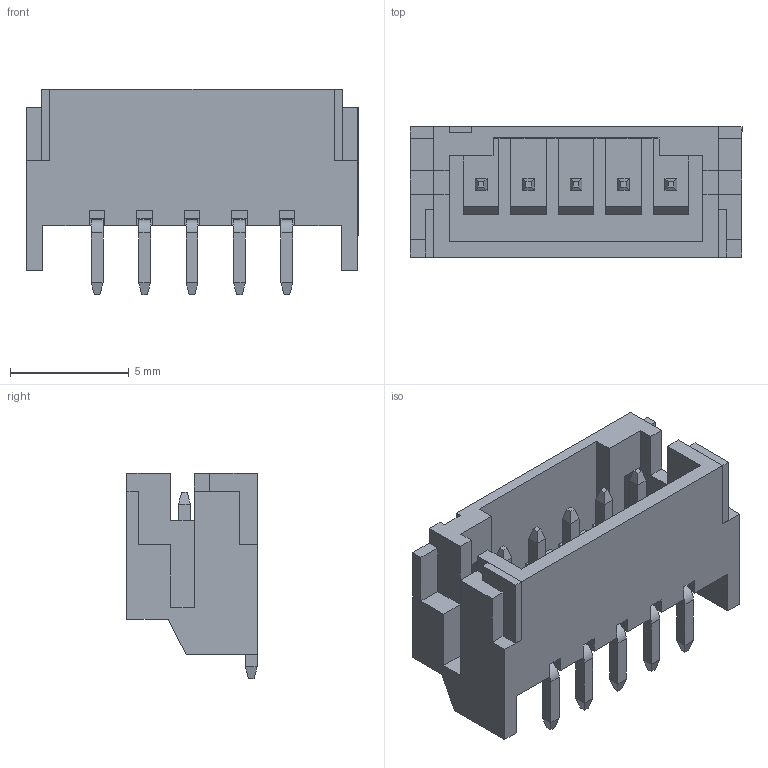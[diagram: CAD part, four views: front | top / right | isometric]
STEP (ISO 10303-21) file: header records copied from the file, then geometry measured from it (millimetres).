
FILE_DESCRIPTION (( 'STEP AP203' ), '1' );
FILE_NAME ('140-505-417-060.STEP', '2020-03-31T20:20:28', ( '' ), ( '' ), 'SwSTEP 2.0', 'SolidWorks 2016', '' );
FILE_SCHEMA (( 'CONFIG_CONTROL_DESIGN' ));
Length unit declared in the file: millimetre
Products named in the file (4): 140-505-417-060; RA SMT Pad; RA SMT Contact; RA SMT Housing_505
Assembly tree (8 placements, depth 2):
  140-505-417-060
    RA SMT Housing_505
    RA SMT Contact  x5
    RA SMT Pad  x2
Bounding box: 14 x 5.5 x 8.65 mm (x, y, z)
Volume: 211.9 mm3; surface area: 768.7 mm2
Topology: 8 solids, 8 shells, 310 faces, 772 edges, 474 vertices
Faces by surface type: plane 290, cylinder 20
Entity records: 6406 total; most frequent: CARTESIAN_POINT 1053, ORIENTED_EDGE 1040, DIRECTION 918, EDGE_CURVE 520, VECTOR 512, LINE 512, VERTEX_POINT 338, AXIS2_PLACEMENT_3D 203
